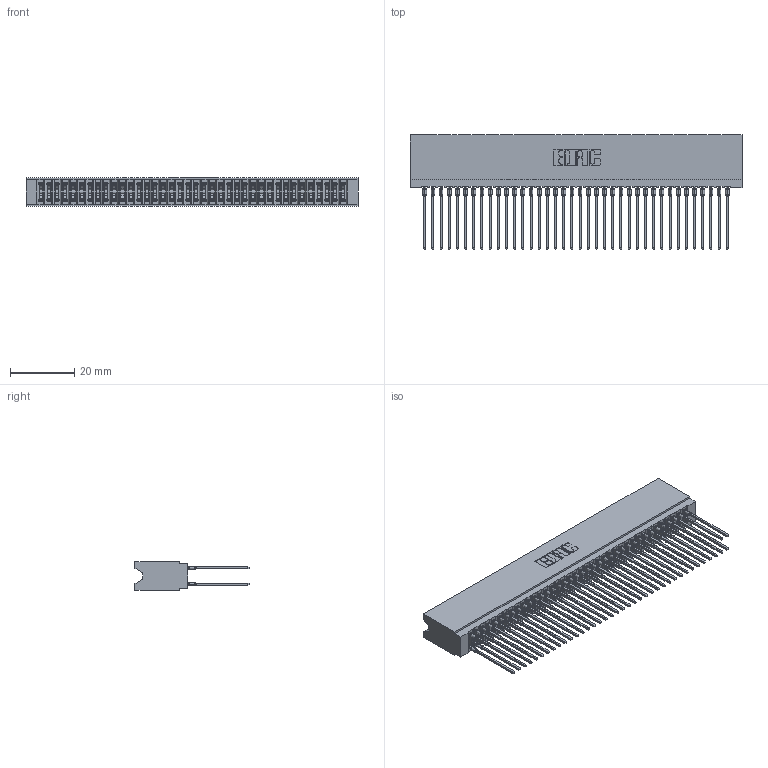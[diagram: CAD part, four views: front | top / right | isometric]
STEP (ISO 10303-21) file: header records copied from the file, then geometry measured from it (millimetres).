
FILE_DESCRIPTION (( 'STEP AP203' ), '1' );
FILE_NAME ('745-076-541-206.STEP', '2026-02-26T20:16:30', ( '' ), ( '' ), 'SwSTEP 2.0', 'SolidWorks 2023', '' );
FILE_SCHEMA (( 'CONFIG_CONTROL_DESIGN' ));
Length unit declared in the file: millimetre
Products named in the file (3): 745-292-001_541; 745 Part_Insulator Option - 06; 745-076-541-206
Assembly tree (77 placements, depth 2):
  745-076-541-206
    745 Part_Insulator Option - 06
    745-292-001_541  x76
Bounding box: 103.12 x 35.45 x 8.89 mm (x, y, z)
Volume: 9661.1 mm3; surface area: 21083.4 mm2
Topology: 77 solids, 77 shells, 6898 faces, 18538 edges, 11648 vertices
Faces by surface type: plane 3552, bspline 1520, cylinder 1370, torus 456
Entity records: 64540 total; most frequent: CARTESIAN_POINT 11698, ORIENTED_EDGE 11126, DIRECTION 9723, EDGE_CURVE 5563, VECTOR 5153, LINE 5153, VERTEX_POINT 3548, AXIS2_PLACEMENT_3D 2285
